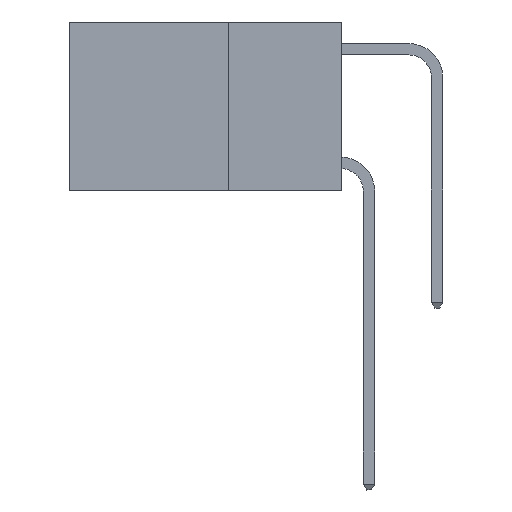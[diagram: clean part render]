
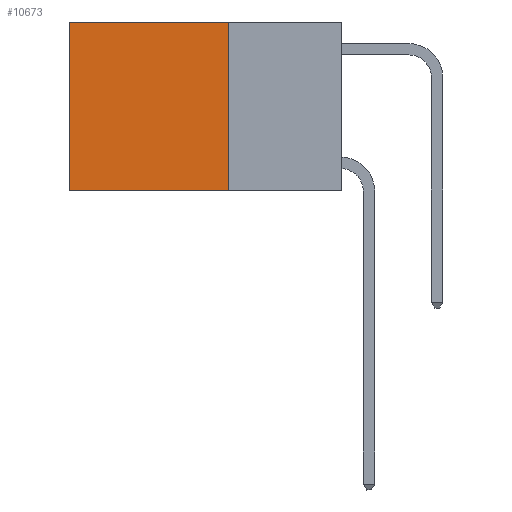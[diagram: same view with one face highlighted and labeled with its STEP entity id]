
A CAD part, left-side view. The second image highlights one B-rep face of the part: STEP entity #10673.
In plain terms, the highlighted planar face has unit normal (-1, 0, 0).
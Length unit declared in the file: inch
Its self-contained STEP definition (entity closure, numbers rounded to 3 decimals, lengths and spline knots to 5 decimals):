
#352 = PLANE ( 'NONE',  #6801 ) ;
#1054 = VERTEX_POINT ( 'NONE', #18786 ) ;
#1060 = LINE ( 'NONE', #14123, #11896 ) ;
#1427 = VERTEX_POINT ( 'NONE', #16954 ) ;
#1647 = ORIENTED_EDGE ( 'NONE', *, *, #9435, .T. ) ;
#1827 = FACE_OUTER_BOUND ( 'NONE', #17200, .T. ) ;
#2259 = VERTEX_POINT ( 'NONE', #6546 ) ;
#3121 = DIRECTION ( 'NONE',  ( 1., 0., 0. ) ) ;
#3704 = DIRECTION ( 'NONE',  ( 0., 1., 0. ) ) ;
#6546 = CARTESIAN_POINT ( 'NONE',  ( 0.2625, 0.6, -0.37 ) ) ;
#6741 = DIRECTION ( 'NONE',  ( 0., 0., -1. ) ) ;
#6801 = AXIS2_PLACEMENT_3D ( 'NONE', #16544, #3121, #10351 ) ;
#6915 = LINE ( 'NONE', #12512, #15657 ) ;
#7922 = DIRECTION ( 'NONE',  ( 0., 0., -1. ) ) ;
#8039 = EDGE_CURVE ( 'NONE', #8232, #1054, #10875, .T. ) ;
#8046 = DIRECTION ( 'NONE',  ( 0., 1., 0. ) ) ;
#8107 = EDGE_CURVE ( 'NONE', #1427, #2259, #1060, .T. ) ;
#8232 = VERTEX_POINT ( 'NONE', #9614 ) ;
#9435 = EDGE_CURVE ( 'NONE', #8232, #1427, #11081, .T. ) ;
#9614 = CARTESIAN_POINT ( 'NONE',  ( 0.2625, 0.25, 0. ) ) ;
#9831 = CARTESIAN_POINT ( 'NONE',  ( 0.2625, 0.25, 0. ) ) ;
#10207 = ORIENTED_EDGE ( 'NONE', *, *, #18580, .F. ) ;
#10351 = DIRECTION ( 'NONE',  ( 0., 0., -1. ) ) ;
#10673 = ADVANCED_FACE ( 'NONE', ( #1827 ), #352, .F. ) ;
#10875 = LINE ( 'NONE', #16676, #15963 ) ;
#11081 = LINE ( 'NONE', #9831, #14940 ) ;
#11896 = VECTOR ( 'NONE', #6741, 39.37008 ) ;
#12512 = CARTESIAN_POINT ( 'NONE',  ( 0.2625, 0.25, -0.37 ) ) ;
#13274 = ORIENTED_EDGE ( 'NONE', *, *, #8039, .F. ) ;
#14123 = CARTESIAN_POINT ( 'NONE',  ( 0.2625, 0.6, 0. ) ) ;
#14940 = VECTOR ( 'NONE', #8046, 39.37008 ) ;
#15474 = ORIENTED_EDGE ( 'NONE', *, *, #8107, .T. ) ;
#15657 = VECTOR ( 'NONE', #3704, 39.37008 ) ;
#15963 = VECTOR ( 'NONE', #7922, 39.37008 ) ;
#16544 = CARTESIAN_POINT ( 'NONE',  ( 0.2625, 0.25, 0. ) ) ;
#16676 = CARTESIAN_POINT ( 'NONE',  ( 0.2625, 0.25, 0. ) ) ;
#16954 = CARTESIAN_POINT ( 'NONE',  ( 0.2625, 0.6, 0. ) ) ;
#17200 = EDGE_LOOP ( 'NONE', ( #15474, #10207, #13274, #1647 ) ) ;
#18580 = EDGE_CURVE ( 'NONE', #1054, #2259, #6915, .T. ) ;
#18786 = CARTESIAN_POINT ( 'NONE',  ( 0.2625, 0.25, -0.37 ) ) ;
